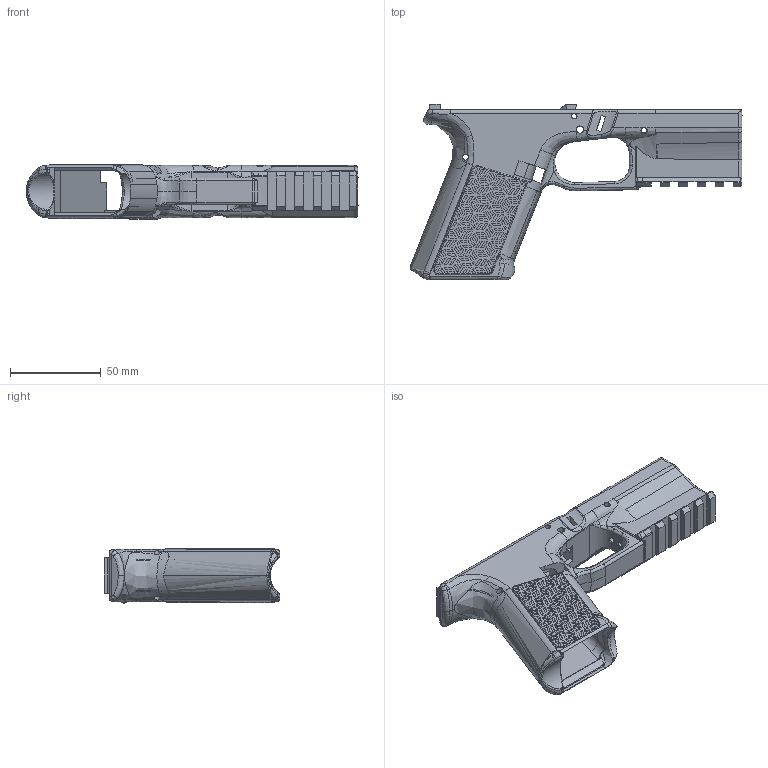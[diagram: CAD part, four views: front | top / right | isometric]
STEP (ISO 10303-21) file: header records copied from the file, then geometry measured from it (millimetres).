
FILE_DESCRIPTION(/* description */ (''),/* implementation_level */ '2;1');
FILE_NAME(/* name */ 'Lil Chungus.step',/* time_stamp */ '2021-04-14T12:58:04-06:00',/* author */ (''),/* organization */ (''),/* preprocessor_version */ 'ST-DEVELOPER v18.1',/* originating_system */ 'Autodesk Translation Framework v10.6.0.1341',/* authorisation */ '');
FILE_SCHEMA (('AUTOMOTIVE_DESIGN { 1 0 10303 214 3 1 1 }'));
Products named in the file (1): Lil Chungus
Bounding box: 183.22 x 97 x 30.34 mm (x, y, z)
Volume: 103203.9 mm3; surface area: 53020 mm2
Topology: 1 solids, 5 shells, 3137 faces, 8471 edges, 5521 vertices
Faces by surface type: plane 1600, bspline 1293, cylinder 187, torus 38, sphere 16, cone 3
Full cylindrical faces by diameter (mm): 2 x1, 3 x6, 3.2 x2, 4 x2, 9.6 x2
Entity records: 124564 total; most frequent: CARTESIAN_POINT 57506, ORIENTED_EDGE 16920, DIRECTION 10184, EDGE_CURVE 8460, VERTEX_POINT 5522, LINE 5194, VECTOR 5194, EDGE_LOOP 3361
